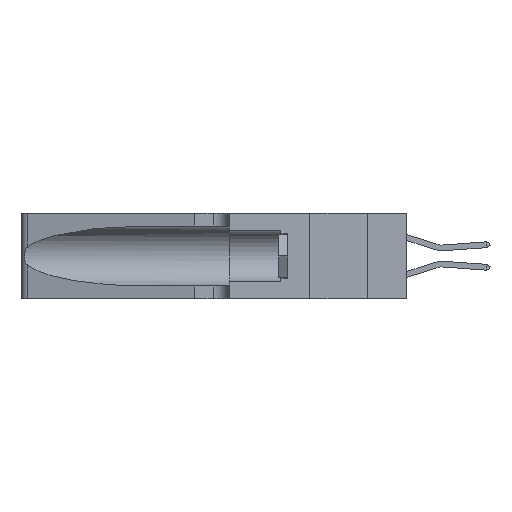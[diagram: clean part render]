
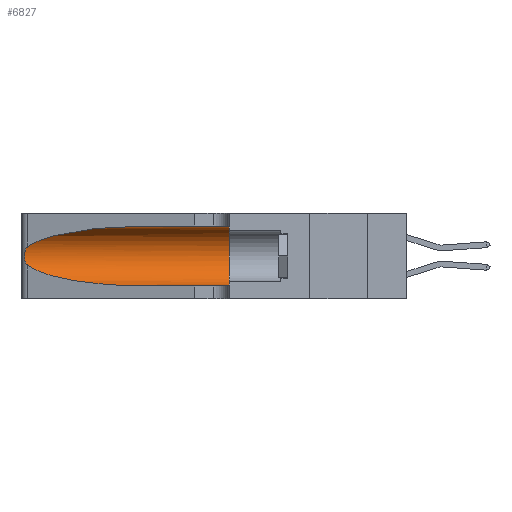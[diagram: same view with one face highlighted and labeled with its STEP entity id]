
A CAD part, left-side view. The second image highlights one B-rep face of the part: STEP entity #6827.
In plain terms, the highlighted cylindrical face has radius 3.308 mm (diameter 6.617 mm), a partial arc.
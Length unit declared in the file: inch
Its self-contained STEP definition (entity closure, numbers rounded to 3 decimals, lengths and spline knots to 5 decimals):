
#566 = CARTESIAN_POINT ( 'NONE',  ( 0.25487, 1.22718, 0.22369 ) ) ;
#671 = CARTESIAN_POINT ( 'NONE',  ( 0.1305, 0.35, 0.05475 ) ) ;
#1769 = CARTESIAN_POINT ( 'NONE',  ( 0.25487, 1.22718, 0.22369 ) ) ;
#1821 = CARTESIAN_POINT ( 'NONE',  ( 0.1305, 0.35, 0.31525 ) ) ;
#1905 = CARTESIAN_POINT ( 'NONE',  ( 0.25639, 1.23186, 0.15144 ) ) ;
#2426 = DIRECTION ( 'NONE',  ( 0., -1., 0. ) ) ;
#3287 = CYLINDRICAL_SURFACE ( 'NONE', #27256, 0.13025 ) ;
#3310 = CARTESIAN_POINT ( 'NONE',  ( 0.25487, 1.22718, 0.14631 ) ) ;
#4117 = ORIENTED_EDGE ( 'NONE', *, *, #30759, .T. ) ;
#5000 = CARTESIAN_POINT ( 'NONE',  ( 0.25487, 1.22718, 0.14631 ) ) ;
#6019 = VERTEX_POINT ( 'NONE', #38218 ) ;
#6365 = DIRECTION ( 'NONE',  ( 0., 1., 0. ) ) ;
#6827 = ADVANCED_FACE ( 'NONE', ( #27533 ), #3287, .F. ) ;
#7820 = VERTEX_POINT ( 'NONE', #1821 ) ;
#8004 = CARTESIAN_POINT ( 'NONE',  ( 0.25639, 1.23184, 0.21858 ) ) ;
#8883 = VERTEX_POINT ( 'NONE', #671 ) ;
#9526 = CARTESIAN_POINT ( 'NONE',  ( 0.1305, 0.72297, 0.05475 ) ) ;
#9552 = CARTESIAN_POINT ( 'NONE',  ( 0.1305, 1.61858, 0.05475 ) ) ;
#9832 = VECTOR ( 'NONE', #21036, 39.37008 ) ;
#11048 = CARTESIAN_POINT ( 'NONE',  ( 0.25854, 1.2359, 0.20912 ) ) ;
#11335 = VERTEX_POINT ( 'NONE', #566 ) ;
#11695 = CARTESIAN_POINT ( 'NONE',  ( 0.1305, 1.61858, 0.185 ) ) ;
#11763 = ORIENTED_EDGE ( 'NONE', *, *, #32828, .T. ) ;
#11849 = CARTESIAN_POINT ( 'NONE',  ( 0.2373, 1.15595, 0.28018 ) ) ;
#13319 = LINE ( 'NONE', #9552, #37332 ) ;
#14116 = CARTESIAN_POINT ( 'NONE',  ( 0.26075, 1.23896, 0.19203 ) ) ;
#16052 = VERTEX_POINT ( 'NONE', #32249 ) ;
#16937 = EDGE_LOOP ( 'NONE', ( #20437, #4117, #25338, #11763, #35198, #17335 ) ) ;
#17164 = CARTESIAN_POINT ( 'NONE',  ( 0.26017, 1.23833, 0.17102 ) ) ;
#17335 = ORIENTED_EDGE ( 'NONE', *, *, #34891, .F. ) ;
#17655 = B_SPLINE_CURVE_WITH_KNOTS ( 'NONE', 3,
 ( #1769, #20062, #8004, #29122, #11048, #32113, #14116, #35134, #17164, #38165, #20188, #1905, #23197, #5000 ),
 .UNSPECIFIED., .F., .F.,
 ( 4, 2, 2, 2, 2, 2, 4 ),
 ( 0., 0.00027, 0.00053, 0.00107, 0.0016, 0.00187, 0.00214 ),
 .UNSPECIFIED. ) ;
#17894 = LINE ( 'NONE', #35998, #9832 ) ;
#18551 = DIRECTION ( 'NONE',  ( 0., -1., 0. ) ) ;
#20062 = CARTESIAN_POINT ( 'NONE',  ( 0.25555, 1.22994, 0.2215 ) ) ;
#20188 = CARTESIAN_POINT ( 'NONE',  ( 0.25789, 1.23486, 0.15765 ) ) ;
#20437 = ORIENTED_EDGE ( 'NONE', *, *, #38447, .T. ) ;
#21036 = DIRECTION ( 'NONE',  ( 0., -1., 0. ) ) ;
#21707 = EDGE_CURVE ( 'NONE', #37383, #6019, #33959, .T. ) ;
#23197 = CARTESIAN_POINT ( 'NONE',  ( 0.25555, 1.22993, 0.14849 ) ) ;
#24509 = CARTESIAN_POINT ( 'NONE',  ( 0.1305, 0.35, 0.185 ) ) ;
#24569 = CARTESIAN_POINT ( 'NONE',  ( 0.2373, 1.15595, 0.08982 ) ) ;
#25338 = ORIENTED_EDGE ( 'NONE', *, *, #21707, .T. ) ;
#25704 = CIRCLE ( 'NONE', #29129, 0.13025 ) ;
#26763 = DIRECTION ( 'NONE',  ( 0., 0., -1. ) ) ;
#26916 = CARTESIAN_POINT ( 'NONE',  ( 0.1305, 0.72297, 0.31525 ) ) ;
#27256 = AXIS2_PLACEMENT_3D ( 'NONE', #11695, #2426, #26763 ) ;
#27533 = FACE_OUTER_BOUND ( 'NONE', #16937, .T. ) ;
#27565 = DIRECTION ( 'NONE',  ( 0., 0., 1. ) ) ;
#27613 = CARTESIAN_POINT ( 'NONE',  ( 0.18966, 0.96281, 0.05475 ) ) ;
#28176 = EDGE_CURVE ( 'NONE', #7820, #8883, #25704, .T. ) ;
#29122 = CARTESIAN_POINT ( 'NONE',  ( 0.25787, 1.23484, 0.2124 ) ) ;
#29129 = AXIS2_PLACEMENT_3D ( 'NONE', #24509, #6365, #27565 ) ;
#29919 = CARTESIAN_POINT ( 'NONE',  ( 0.18966, 0.96281, 0.31525 ) ) ;
#30759 = EDGE_CURVE ( 'NONE', #11335, #37383, #17655, .T. ) ;
#32113 = CARTESIAN_POINT ( 'NONE',  ( 0.26018, 1.23835, 0.19895 ) ) ;
#32249 = CARTESIAN_POINT ( 'NONE',  ( 0.1305, 0.72297, 0.31525 ) ) ;
#32287 = CARTESIAN_POINT ( 'NONE',  ( 0.25487, 1.22718, 0.14631 ) ) ;
#32828 = EDGE_CURVE ( 'NONE', #6019, #8883, #13319, .T. ) ;
#32922 = CARTESIAN_POINT ( 'NONE',  ( 0.25487, 1.22718, 0.22369 ) ) ;
#33959 =( BOUNDED_CURVE ( )  B_SPLINE_CURVE ( 3, ( #3310, #24569, #27613, #9526 ),
 .UNSPECIFIED., .F., .T. ) 
 B_SPLINE_CURVE_WITH_KNOTS ( ( 4, 4 ),
 ( 3.44316, 4.71239 ),
 .UNSPECIFIED. ) 
 CURVE ( )  GEOMETRIC_REPRESENTATION_ITEM ( )  RATIONAL_B_SPLINE_CURVE ( ( 1., 0.87, 0.87, 1. ) ) 
 REPRESENTATION_ITEM ( '' )  );
#34837 =( BOUNDED_CURVE ( )  B_SPLINE_CURVE ( 3, ( #26916, #29919, #11849, #32922 ),
 .UNSPECIFIED., .F., .F. ) 
 B_SPLINE_CURVE_WITH_KNOTS ( ( 4, 4 ),
 ( 1.5708, 2.84003 ),
 .UNSPECIFIED. ) 
 CURVE ( )  GEOMETRIC_REPRESENTATION_ITEM ( )  RATIONAL_B_SPLINE_CURVE ( ( 1., 0.87, 0.87, 1. ) ) 
 REPRESENTATION_ITEM ( '' )  );
#34891 = EDGE_CURVE ( 'NONE', #16052, #7820, #17894, .T. ) ;
#35134 = CARTESIAN_POINT ( 'NONE',  ( 0.26075, 1.23896, 0.178 ) ) ;
#35198 = ORIENTED_EDGE ( 'NONE', *, *, #28176, .F. ) ;
#35998 = CARTESIAN_POINT ( 'NONE',  ( 0.1305, 1.61858, 0.31525 ) ) ;
#37332 = VECTOR ( 'NONE', #18551, 39.37008 ) ;
#37383 = VERTEX_POINT ( 'NONE', #32287 ) ;
#38165 = CARTESIAN_POINT ( 'NONE',  ( 0.25856, 1.23593, 0.16098 ) ) ;
#38218 = CARTESIAN_POINT ( 'NONE',  ( 0.1305, 0.72297, 0.05475 ) ) ;
#38447 = EDGE_CURVE ( 'NONE', #16052, #11335, #34837, .T. ) ;
